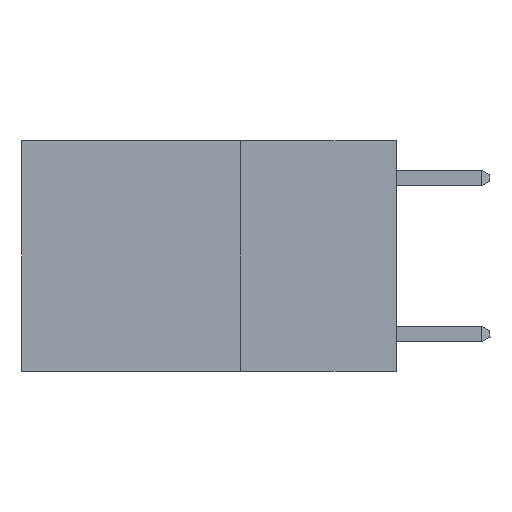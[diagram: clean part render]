
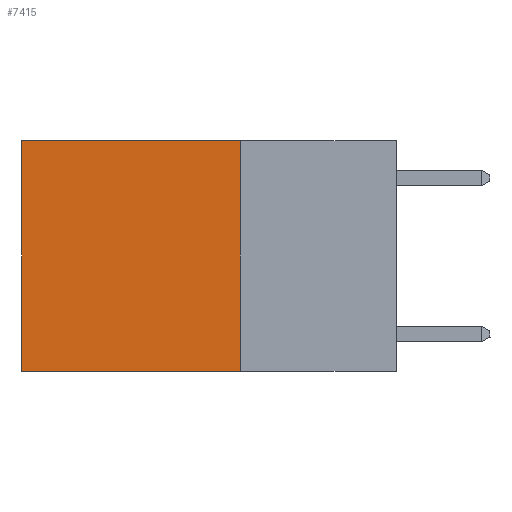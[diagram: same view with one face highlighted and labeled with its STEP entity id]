
A CAD part, left-side view. The second image highlights one B-rep face of the part: STEP entity #7415.
In plain terms, the highlighted planar face has unit normal (-1, 0, 0).
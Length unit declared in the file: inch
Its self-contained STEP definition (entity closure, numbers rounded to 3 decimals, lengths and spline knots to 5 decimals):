
#919 = DIRECTION ( 'NONE',  ( 1., 0., 0. ) ) ;
#1144 = EDGE_CURVE ( 'NONE', #8217, #4226, #17707, .T. ) ;
#1944 = VECTOR ( 'NONE', #10957, 39.37008 ) ;
#2033 = EDGE_CURVE ( 'NONE', #11521, #8217, #14188, .T. ) ;
#2953 = FACE_OUTER_BOUND ( 'NONE', #12471, .T. ) ;
#3773 = VECTOR ( 'NONE', #8846, 39.37008 ) ;
#4226 = VERTEX_POINT ( 'NONE', #13756 ) ;
#5082 = DIRECTION ( 'NONE',  ( 0., 0., -1. ) ) ;
#5432 = PLANE ( 'NONE',  #6517 ) ;
#5856 = CARTESIAN_POINT ( 'NONE',  ( 0.2625, 0.6, 0. ) ) ;
#6517 = AXIS2_PLACEMENT_3D ( 'NONE', #9835, #919, #11259 ) ;
#7232 = ORIENTED_EDGE ( 'NONE', *, *, #9998, .T. ) ;
#7257 = CARTESIAN_POINT ( 'NONE',  ( 0.2625, 0.25, -0.37 ) ) ;
#7415 = ADVANCED_FACE ( 'NONE', ( #2953 ), #5432, .F. ) ;
#8217 = VERTEX_POINT ( 'NONE', #7257 ) ;
#8846 = DIRECTION ( 'NONE',  ( 0., 0., -1. ) ) ;
#9835 = CARTESIAN_POINT ( 'NONE',  ( 0.2625, 0.25, 0. ) ) ;
#9998 = EDGE_CURVE ( 'NONE', #11521, #16135, #14137, .T. ) ;
#10134 = ORIENTED_EDGE ( 'NONE', *, *, #10159, .T. ) ;
#10159 = EDGE_CURVE ( 'NONE', #16135, #4226, #15234, .T. ) ;
#10426 = VECTOR ( 'NONE', #16930, 39.37008 ) ;
#10578 = ORIENTED_EDGE ( 'NONE', *, *, #1144, .F. ) ;
#10957 = DIRECTION ( 'NONE',  ( 0., 1., 0. ) ) ;
#11259 = DIRECTION ( 'NONE',  ( 0., 0., -1. ) ) ;
#11521 = VERTEX_POINT ( 'NONE', #14672 ) ;
#12471 = EDGE_LOOP ( 'NONE', ( #10134, #10578, #14291, #7232 ) ) ;
#13756 = CARTESIAN_POINT ( 'NONE',  ( 0.2625, 0.6, -0.37 ) ) ;
#14137 = LINE ( 'NONE', #15539, #10426 ) ;
#14188 = LINE ( 'NONE', #15070, #17441 ) ;
#14291 = ORIENTED_EDGE ( 'NONE', *, *, #2033, .F. ) ;
#14672 = CARTESIAN_POINT ( 'NONE',  ( 0.2625, 0.25, 0. ) ) ;
#15070 = CARTESIAN_POINT ( 'NONE',  ( 0.2625, 0.25, 0. ) ) ;
#15234 = LINE ( 'NONE', #5856, #3773 ) ;
#15539 = CARTESIAN_POINT ( 'NONE',  ( 0.2625, 0.25, 0. ) ) ;
#15896 = CARTESIAN_POINT ( 'NONE',  ( 0.2625, 0.6, 0. ) ) ;
#16135 = VERTEX_POINT ( 'NONE', #15896 ) ;
#16930 = DIRECTION ( 'NONE',  ( 0., 1., 0. ) ) ;
#17441 = VECTOR ( 'NONE', #5082, 39.37008 ) ;
#17707 = LINE ( 'NONE', #17920, #1944 ) ;
#17920 = CARTESIAN_POINT ( 'NONE',  ( 0.2625, 0.25, -0.37 ) ) ;
